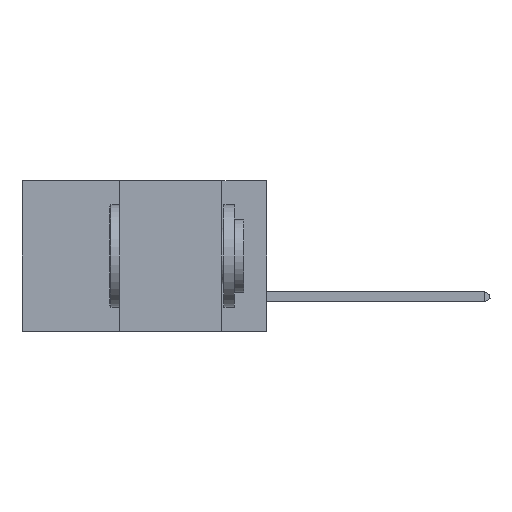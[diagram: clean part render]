
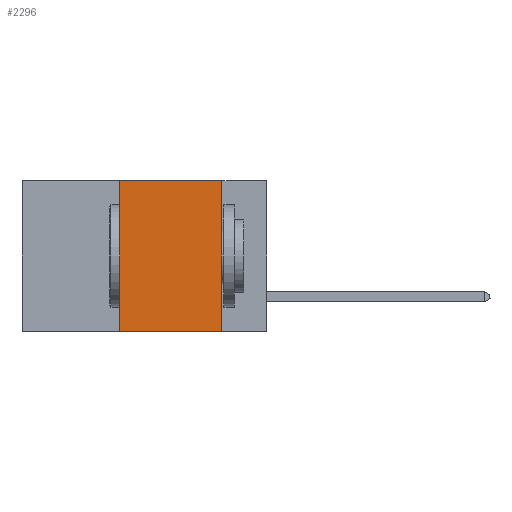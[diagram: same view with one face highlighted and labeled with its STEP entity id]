
A CAD part, left-side view. The second image highlights one B-rep face of the part: STEP entity #2296.
In plain terms, the highlighted planar face has unit normal (-1, 0, 0).
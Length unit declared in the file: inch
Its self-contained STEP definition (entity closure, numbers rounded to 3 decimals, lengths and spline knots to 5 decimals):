
#213 = DIRECTION ( 'NONE',  ( 1., 0., 0. ) ) ;
#522 = CARTESIAN_POINT ( 'NONE',  ( 0., 0.11, 0. ) ) ;
#741 = CARTESIAN_POINT ( 'NONE',  ( 0., 0.11, 0. ) ) ;
#1225 = CARTESIAN_POINT ( 'NONE',  ( 0., 0.6, -0.37 ) ) ;
#1454 = EDGE_CURVE ( 'NONE', #7938, #5836, #11123, .T. ) ;
#1744 = FACE_OUTER_BOUND ( 'NONE', #3567, .T. ) ;
#1952 = DIRECTION ( 'NONE',  ( 0., 0., -1. ) ) ;
#2296 = ADVANCED_FACE ( 'NONE', ( #1744 ), #3496, .F. ) ;
#3150 = VERTEX_POINT ( 'NONE', #522 ) ;
#3496 = PLANE ( 'NONE',  #3499 ) ;
#3499 = AXIS2_PLACEMENT_3D ( 'NONE', #8810, #213, #1952 ) ;
#3567 = EDGE_LOOP ( 'NONE', ( #6881, #6916, #6252, #5298 ) ) ;
#3699 = CARTESIAN_POINT ( 'NONE',  ( 0., 0.6, 0. ) ) ;
#4346 = DIRECTION ( 'NONE',  ( 0., 0., -1. ) ) ;
#4388 = LINE ( 'NONE', #741, #7279 ) ;
#4392 = VECTOR ( 'NONE', #9562, 39.37008 ) ;
#5298 = ORIENTED_EDGE ( 'NONE', *, *, #1454, .T. ) ;
#5836 = VERTEX_POINT ( 'NONE', #7921 ) ;
#5942 = CARTESIAN_POINT ( 'NONE',  ( 0., 0.36, 0. ) ) ;
#6129 = VERTEX_POINT ( 'NONE', #5942 ) ;
#6252 = ORIENTED_EDGE ( 'NONE', *, *, #11358, .F. ) ;
#6429 = DIRECTION ( 'NONE',  ( 0., -1., 0. ) ) ;
#6481 = LINE ( 'NONE', #7040, #4392 ) ;
#6528 = VECTOR ( 'NONE', #6429, 39.37008 ) ;
#6720 = VECTOR ( 'NONE', #7362, 39.37008 ) ;
#6881 = ORIENTED_EDGE ( 'NONE', *, *, #8265, .F. ) ;
#6916 = ORIENTED_EDGE ( 'NONE', *, *, #9727, .F. ) ;
#7032 = CARTESIAN_POINT ( 'NONE',  ( 0., 0.36, -0.37 ) ) ;
#7040 = CARTESIAN_POINT ( 'NONE',  ( 0., 0.36, 0. ) ) ;
#7279 = VECTOR ( 'NONE', #4346, 39.37008 ) ;
#7362 = DIRECTION ( 'NONE',  ( 0., -1., 0. ) ) ;
#7921 = CARTESIAN_POINT ( 'NONE',  ( 0., 0.11, -0.37 ) ) ;
#7938 = VERTEX_POINT ( 'NONE', #7032 ) ;
#8265 = EDGE_CURVE ( 'NONE', #3150, #5836, #4388, .T. ) ;
#8810 = CARTESIAN_POINT ( 'NONE',  ( 0., 0.6, 0. ) ) ;
#9562 = DIRECTION ( 'NONE',  ( 0., 0., 1. ) ) ;
#9727 = EDGE_CURVE ( 'NONE', #6129, #3150, #10349, .T. ) ;
#10349 = LINE ( 'NONE', #3699, #6528 ) ;
#11123 = LINE ( 'NONE', #1225, #6720 ) ;
#11358 = EDGE_CURVE ( 'NONE', #7938, #6129, #6481, .T. ) ;
